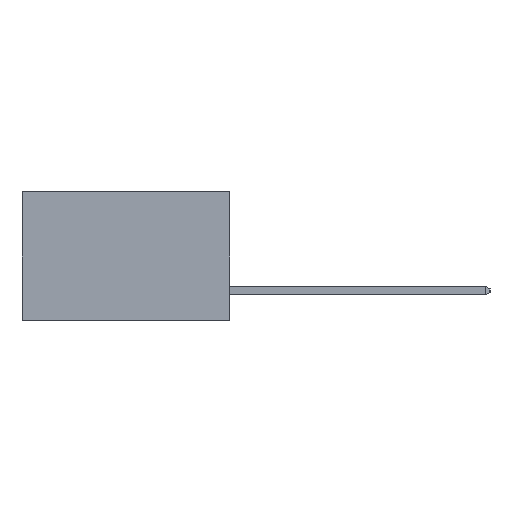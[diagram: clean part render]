
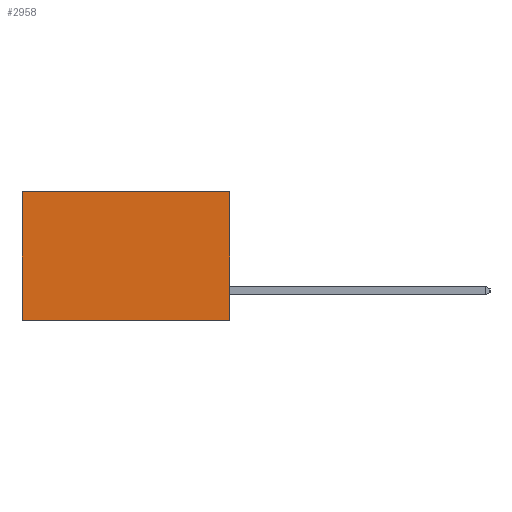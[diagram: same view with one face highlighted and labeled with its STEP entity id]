
A CAD part, left-side view. The second image highlights one B-rep face of the part: STEP entity #2958.
In plain terms, the highlighted planar face has unit normal (-1, 0, 0).
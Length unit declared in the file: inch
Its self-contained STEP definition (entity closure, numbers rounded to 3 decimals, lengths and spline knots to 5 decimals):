
#79 = LINE ( 'NONE', #7094, #3089 ) ;
#116 = CARTESIAN_POINT ( 'NONE',  ( 0.2615, 0.6, -0.37 ) ) ;
#366 = EDGE_CURVE ( 'NONE', #3118, #6796, #4704, .T. ) ;
#625 = VERTEX_POINT ( 'NONE', #783 ) ;
#646 = CARTESIAN_POINT ( 'NONE',  ( 0.2615, 0., 0. ) ) ;
#665 = ORIENTED_EDGE ( 'NONE', *, *, #3745, .F. ) ;
#783 = CARTESIAN_POINT ( 'NONE',  ( 0.2615, 0.6, 0. ) ) ;
#988 = VECTOR ( 'NONE', #1224, 39.37008 ) ;
#1224 = DIRECTION ( 'NONE',  ( 0., 0., -1. ) ) ;
#1936 = VECTOR ( 'NONE', #10201, 39.37008 ) ;
#2579 = CARTESIAN_POINT ( 'NONE',  ( 0.2615, 0., -0.37 ) ) ;
#2775 = EDGE_LOOP ( 'NONE', ( #9900, #665, #3343, #10135 ) ) ;
#2958 = ADVANCED_FACE ( 'NONE', ( #8607 ), #5208, .F. ) ;
#3089 = VECTOR ( 'NONE', #7116, 39.37008 ) ;
#3118 = VERTEX_POINT ( 'NONE', #646 ) ;
#3343 = ORIENTED_EDGE ( 'NONE', *, *, #366, .F. ) ;
#3745 = EDGE_CURVE ( 'NONE', #6796, #3913, #10918, .T. ) ;
#3913 = VERTEX_POINT ( 'NONE', #4120 ) ;
#3979 = CARTESIAN_POINT ( 'NONE',  ( 0.2615, 0., -0.37 ) ) ;
#4120 = CARTESIAN_POINT ( 'NONE',  ( 0.2615, 0.6, -0.37 ) ) ;
#4500 = EDGE_CURVE ( 'NONE', #3118, #625, #79, .T. ) ;
#4691 = VECTOR ( 'NONE', #7612, 39.37008 ) ;
#4704 = LINE ( 'NONE', #3979, #988 ) ;
#4956 = LINE ( 'NONE', #116, #4691 ) ;
#5208 = PLANE ( 'NONE',  #10613 ) ;
#6466 = DIRECTION ( 'NONE',  ( 0., 0., -1. ) ) ;
#6770 = EDGE_CURVE ( 'NONE', #625, #3913, #4956, .T. ) ;
#6781 = DIRECTION ( 'NONE',  ( 1., 0., 0. ) ) ;
#6796 = VERTEX_POINT ( 'NONE', #8426 ) ;
#7094 = CARTESIAN_POINT ( 'NONE',  ( 0.2615, 0., 0. ) ) ;
#7116 = DIRECTION ( 'NONE',  ( 0., 1., 0. ) ) ;
#7612 = DIRECTION ( 'NONE',  ( 0., 0., -1. ) ) ;
#8426 = CARTESIAN_POINT ( 'NONE',  ( 0.2615, 0., -0.37 ) ) ;
#8607 = FACE_OUTER_BOUND ( 'NONE', #2775, .T. ) ;
#9900 = ORIENTED_EDGE ( 'NONE', *, *, #6770, .T. ) ;
#10135 = ORIENTED_EDGE ( 'NONE', *, *, #4500, .T. ) ;
#10201 = DIRECTION ( 'NONE',  ( 0., 1., 0. ) ) ;
#10233 = CARTESIAN_POINT ( 'NONE',  ( 0.2615, 0., -0.37 ) ) ;
#10613 = AXIS2_PLACEMENT_3D ( 'NONE', #2579, #6781, #6466 ) ;
#10918 = LINE ( 'NONE', #10233, #1936 ) ;
